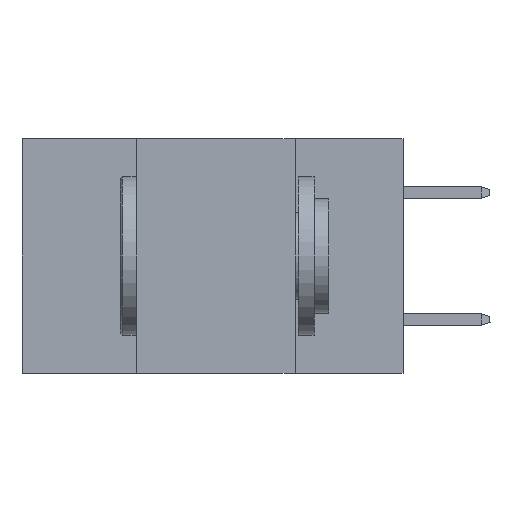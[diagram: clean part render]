
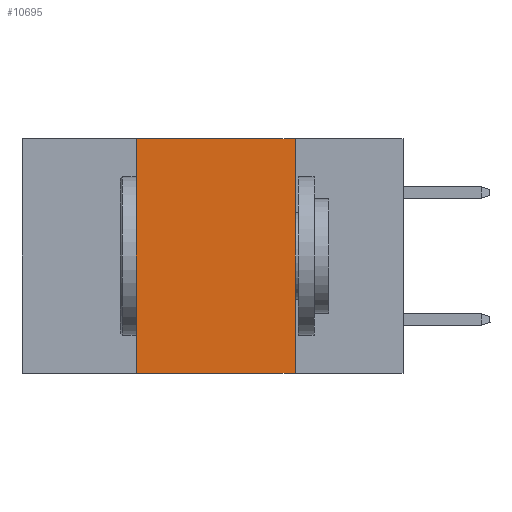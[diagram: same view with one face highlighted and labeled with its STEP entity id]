
A CAD part, left-side view. The second image highlights one B-rep face of the part: STEP entity #10695.
In plain terms, the highlighted planar face has unit normal (-1, 0, 0).
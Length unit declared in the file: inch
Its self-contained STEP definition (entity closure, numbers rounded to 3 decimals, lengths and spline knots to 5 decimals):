
#945 = DIRECTION ( 'NONE',  ( 1., 0., 0. ) ) ;
#1322 = CARTESIAN_POINT ( 'NONE',  ( 0., 0.6, 0. ) ) ;
#1636 = CARTESIAN_POINT ( 'NONE',  ( 0., 0.17, -0.37 ) ) ;
#1833 = DIRECTION ( 'NONE',  ( 0., 0., -1. ) ) ;
#1924 = LINE ( 'NONE', #3224, #12459 ) ;
#2028 = ORIENTED_EDGE ( 'NONE', *, *, #7370, .F. ) ;
#2955 = ORIENTED_EDGE ( 'NONE', *, *, #7705, .T. ) ;
#3085 = PLANE ( 'NONE',  #3816 ) ;
#3224 = CARTESIAN_POINT ( 'NONE',  ( 0., 0.6, -0.37 ) ) ;
#3469 = DIRECTION ( 'NONE',  ( 0., -1., 0. ) ) ;
#3816 = AXIS2_PLACEMENT_3D ( 'NONE', #6574, #945, #8961 ) ;
#4465 = DIRECTION ( 'NONE',  ( 0., -1., 0. ) ) ;
#4676 = ORIENTED_EDGE ( 'NONE', *, *, #10627, .F. ) ;
#4819 = VERTEX_POINT ( 'NONE', #10011 ) ;
#5359 = CARTESIAN_POINT ( 'NONE',  ( 0., 0.17, 0. ) ) ;
#5677 = LINE ( 'NONE', #1322, #10520 ) ;
#6448 = VERTEX_POINT ( 'NONE', #12834 ) ;
#6487 = VERTEX_POINT ( 'NONE', #13356 ) ;
#6574 = CARTESIAN_POINT ( 'NONE',  ( 0., 0.6, 0. ) ) ;
#7370 = EDGE_CURVE ( 'NONE', #4819, #6448, #5677, .T. ) ;
#7705 = EDGE_CURVE ( 'NONE', #6487, #10295, #1924, .T. ) ;
#8714 = EDGE_CURVE ( 'NONE', #6448, #10295, #13420, .T. ) ;
#8799 = LINE ( 'NONE', #13366, #13941 ) ;
#8961 = DIRECTION ( 'NONE',  ( 0., 0., -1. ) ) ;
#9596 = EDGE_LOOP ( 'NONE', ( #13909, #2028, #4676, #2955 ) ) ;
#10011 = CARTESIAN_POINT ( 'NONE',  ( 0., 0.42, 0. ) ) ;
#10295 = VERTEX_POINT ( 'NONE', #1636 ) ;
#10520 = VECTOR ( 'NONE', #3469, 39.37008 ) ;
#10627 = EDGE_CURVE ( 'NONE', #6487, #4819, #8799, .T. ) ;
#10695 = ADVANCED_FACE ( 'NONE', ( #11489 ), #3085, .F. ) ;
#11489 = FACE_OUTER_BOUND ( 'NONE', #9596, .T. ) ;
#12087 = DIRECTION ( 'NONE',  ( 0., 0., 1. ) ) ;
#12222 = VECTOR ( 'NONE', #1833, 39.37008 ) ;
#12459 = VECTOR ( 'NONE', #4465, 39.37008 ) ;
#12834 = CARTESIAN_POINT ( 'NONE',  ( 0., 0.17, 0. ) ) ;
#13356 = CARTESIAN_POINT ( 'NONE',  ( 0., 0.42, -0.37 ) ) ;
#13366 = CARTESIAN_POINT ( 'NONE',  ( 0., 0.42, 0. ) ) ;
#13420 = LINE ( 'NONE', #5359, #12222 ) ;
#13909 = ORIENTED_EDGE ( 'NONE', *, *, #8714, .F. ) ;
#13941 = VECTOR ( 'NONE', #12087, 39.37008 ) ;
